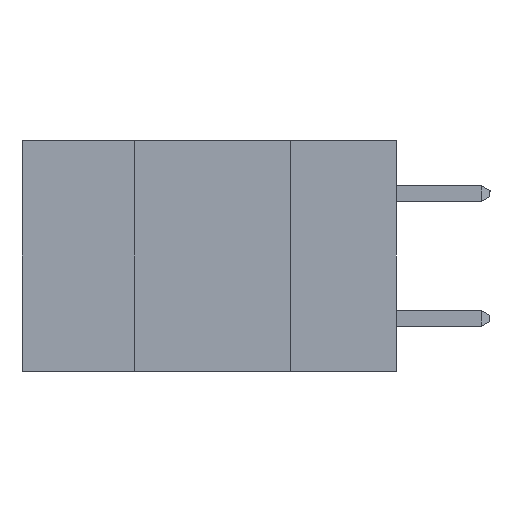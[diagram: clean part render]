
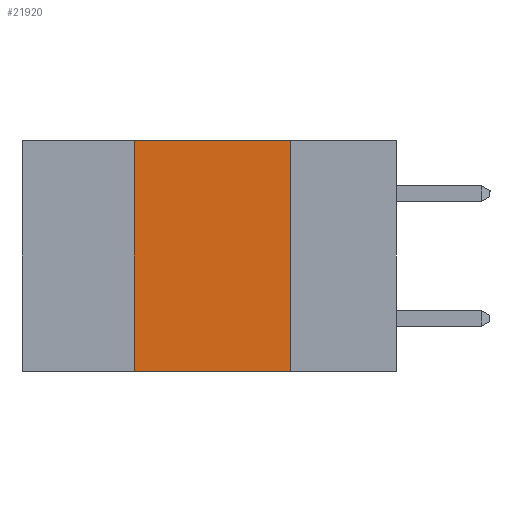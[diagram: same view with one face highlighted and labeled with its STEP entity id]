
A CAD part, left-side view. The second image highlights one B-rep face of the part: STEP entity #21920.
In plain terms, the highlighted planar face has unit normal (-1, 0, 0).
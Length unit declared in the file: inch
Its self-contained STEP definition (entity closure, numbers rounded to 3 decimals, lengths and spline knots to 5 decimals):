
#295 = DIRECTION ( 'NONE',  ( 1., 0., 0. ) ) ;
#322 = CARTESIAN_POINT ( 'NONE',  ( 0., 0.42, -0.37 ) ) ;
#424 = EDGE_CURVE ( 'NONE', #2943, #12897, #12769, .T. ) ;
#2943 = VERTEX_POINT ( 'NONE', #322 ) ;
#3053 = DIRECTION ( 'NONE',  ( 0., -1., 0. ) ) ;
#5352 = LINE ( 'NONE', #16723, #8239 ) ;
#6010 = FACE_OUTER_BOUND ( 'NONE', #15330, .T. ) ;
#6242 = ORIENTED_EDGE ( 'NONE', *, *, #424, .T. ) ;
#6428 = ORIENTED_EDGE ( 'NONE', *, *, #18454, .F. ) ;
#6671 = VECTOR ( 'NONE', #3053, 39.37008 ) ;
#7344 = VECTOR ( 'NONE', #20607, 39.37008 ) ;
#7371 = LINE ( 'NONE', #9126, #7344 ) ;
#8239 = VECTOR ( 'NONE', #22572, 39.37008 ) ;
#9126 = CARTESIAN_POINT ( 'NONE',  ( 0., 0.42, -0.37 ) ) ;
#10378 = CARTESIAN_POINT ( 'NONE',  ( 0., 0.42, 0. ) ) ;
#10562 = DIRECTION ( 'NONE',  ( 0., -1., 0. ) ) ;
#12457 = VECTOR ( 'NONE', #10562, 39.37008 ) ;
#12574 = EDGE_CURVE ( 'NONE', #23531, #12897, #5352, .T. ) ;
#12769 = LINE ( 'NONE', #18401, #6671 ) ;
#12897 = VERTEX_POINT ( 'NONE', #14203 ) ;
#12901 = AXIS2_PLACEMENT_3D ( 'NONE', #17398, #295, #19618 ) ;
#14203 = CARTESIAN_POINT ( 'NONE',  ( 0., 0.17, -0.37 ) ) ;
#15246 = ORIENTED_EDGE ( 'NONE', *, *, #12574, .F. ) ;
#15330 = EDGE_LOOP ( 'NONE', ( #15246, #6428, #24599, #6242 ) ) ;
#15365 = VERTEX_POINT ( 'NONE', #10378 ) ;
#16723 = CARTESIAN_POINT ( 'NONE',  ( 0., 0.17, -0.37 ) ) ;
#17398 = CARTESIAN_POINT ( 'NONE',  ( 0., 0.6, 0. ) ) ;
#17597 = CARTESIAN_POINT ( 'NONE',  ( 0., 0.17, 0. ) ) ;
#18401 = CARTESIAN_POINT ( 'NONE',  ( 0., 0.6, -0.37 ) ) ;
#18454 = EDGE_CURVE ( 'NONE', #15365, #23531, #19928, .T. ) ;
#19618 = DIRECTION ( 'NONE',  ( 0., 0., -1. ) ) ;
#19928 = LINE ( 'NONE', #23535, #12457 ) ;
#20607 = DIRECTION ( 'NONE',  ( 0., 0., 1. ) ) ;
#21494 = PLANE ( 'NONE',  #12901 ) ;
#21920 = ADVANCED_FACE ( 'NONE', ( #6010 ), #21494, .F. ) ;
#22145 = EDGE_CURVE ( 'NONE', #2943, #15365, #7371, .T. ) ;
#22572 = DIRECTION ( 'NONE',  ( 0., 0., -1. ) ) ;
#23531 = VERTEX_POINT ( 'NONE', #17597 ) ;
#23535 = CARTESIAN_POINT ( 'NONE',  ( 0., 0.6, 0. ) ) ;
#24599 = ORIENTED_EDGE ( 'NONE', *, *, #22145, .F. ) ;
